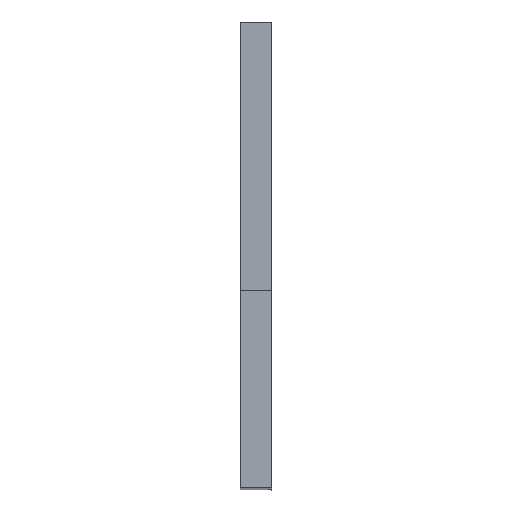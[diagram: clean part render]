
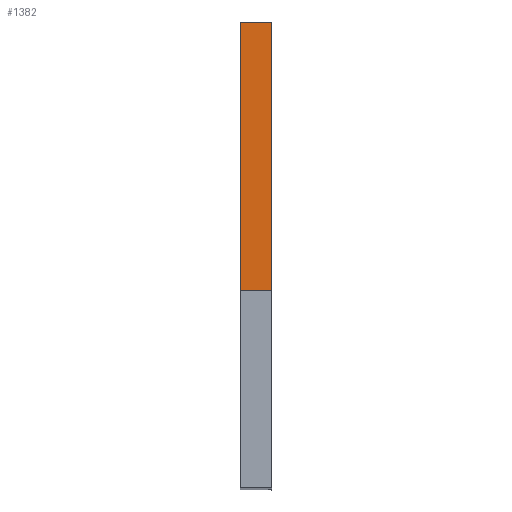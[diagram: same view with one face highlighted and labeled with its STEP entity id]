
A CAD part, top view. The second image highlights one B-rep face of the part: STEP entity #1382.
In plain terms, the highlighted planar face has unit normal (0, 0, 1).
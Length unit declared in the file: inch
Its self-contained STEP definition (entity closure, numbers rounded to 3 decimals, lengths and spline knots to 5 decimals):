
#59=PLANE('',#1497);
#129=FACE_OUTER_BOUND('',#225,.T.);
#225=EDGE_LOOP('',(#1244,#1245,#1246,#1247));
#400=LINE('',#2743,#484);
#415=LINE('',#3547,#499);
#431=LINE('',#4456,#515);
#432=LINE('',#4457,#516);
#484=VECTOR('',#1661,0.3937);
#499=VECTOR('',#1702,0.3937);
#515=VECTOR('',#1776,0.3937);
#516=VECTOR('',#1777,0.3937);
#621=VERTEX_POINT('',#2740);
#622=VERTEX_POINT('',#2742);
#643=VERTEX_POINT('',#3544);
#644=VERTEX_POINT('',#3546);
#780=EDGE_CURVE('',#621,#622,#400,.T.);
#819=EDGE_CURVE('',#643,#644,#415,.T.);
#857=EDGE_CURVE('',#643,#622,#431,.T.);
#858=EDGE_CURVE('',#644,#621,#432,.T.);
#1244=ORIENTED_EDGE('',*,*,#819,.F.);
#1245=ORIENTED_EDGE('',*,*,#857,.T.);
#1246=ORIENTED_EDGE('',*,*,#780,.F.);
#1247=ORIENTED_EDGE('',*,*,#858,.F.);
#1382=ADVANCED_FACE('',(#129),#59,.T.);
#1497=AXIS2_PLACEMENT_3D('',#4455,#1774,#1775);
#1661=DIRECTION('',(0.,1.,0.));
#1702=DIRECTION('',(0.,-1.,0.));
#1774=DIRECTION('center_axis',(0.,0.,1.));
#1775=DIRECTION('ref_axis',(0.,1.,0.));
#1776=DIRECTION('',(-1.,0.,0.));
#1777=DIRECTION('',(-1.,0.,0.));
#2740=CARTESIAN_POINT('',(-0.453,-0.768,0.285));
#2742=CARTESIAN_POINT('',(-0.453,0.,0.285));
#2743=CARTESIAN_POINT('',(-0.453,-0.718,0.285));
#3544=CARTESIAN_POINT('',(-0.363,0.,0.285));
#3546=CARTESIAN_POINT('',(-0.363,-0.768,0.285));
#3547=CARTESIAN_POINT('',(-0.363,-0.718,0.285));
#4455=CARTESIAN_POINT('Origin',(-0.363,-0.768,0.285));
#4456=CARTESIAN_POINT('',(-0.363,0.,0.285));
#4457=CARTESIAN_POINT('',(-0.363,-0.768,0.285));
